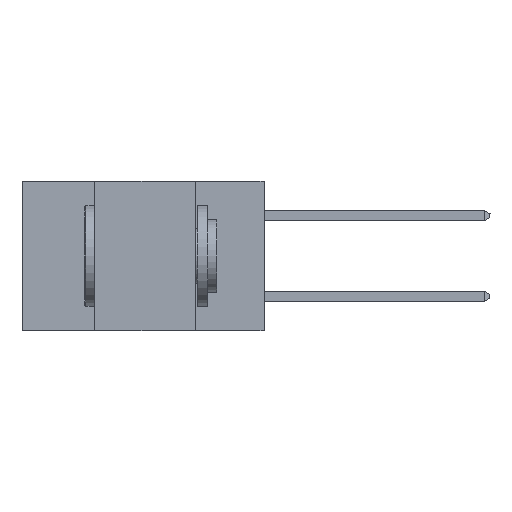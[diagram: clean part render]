
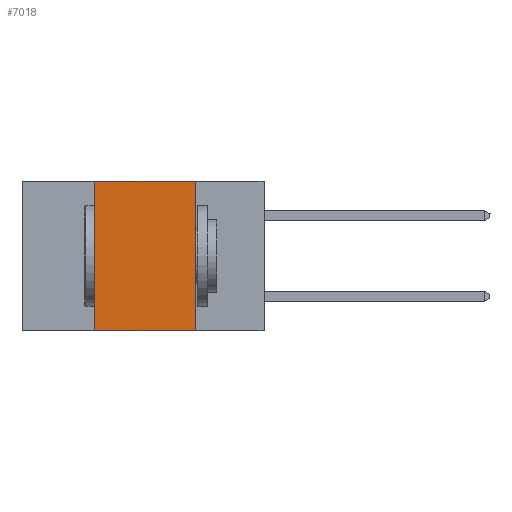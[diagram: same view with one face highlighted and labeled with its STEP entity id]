
A CAD part, left-side view. The second image highlights one B-rep face of the part: STEP entity #7018.
In plain terms, the highlighted planar face has unit normal (-1, 0, 0).
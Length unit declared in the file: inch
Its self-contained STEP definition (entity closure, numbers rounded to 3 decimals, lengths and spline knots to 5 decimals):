
#452 = VERTEX_POINT ( 'NONE', #6241 ) ;
#821 = CARTESIAN_POINT ( 'NONE',  ( 0., 0.42, 0. ) ) ;
#1814 = VECTOR ( 'NONE', #8609, 39.37008 ) ;
#2559 = DIRECTION ( 'NONE',  ( 0., 0., 1. ) ) ;
#2739 = VERTEX_POINT ( 'NONE', #3098 ) ;
#3098 = CARTESIAN_POINT ( 'NONE',  ( 0., 0.17, -0.37 ) ) ;
#3528 = EDGE_LOOP ( 'NONE', ( #12160, #8300, #13146, #19462 ) ) ;
#3588 = CARTESIAN_POINT ( 'NONE',  ( 0., 0.6, 0. ) ) ;
#6241 = CARTESIAN_POINT ( 'NONE',  ( 0., 0.42, 0. ) ) ;
#6945 = CARTESIAN_POINT ( 'NONE',  ( 0., 0.6, 0. ) ) ;
#7010 = DIRECTION ( 'NONE',  ( 1., 0., 0. ) ) ;
#7018 = ADVANCED_FACE ( 'NONE', ( #9118 ), #16418, .F. ) ;
#7103 = CARTESIAN_POINT ( 'NONE',  ( 0., 0.17, 0. ) ) ;
#7182 = LINE ( 'NONE', #19060, #18537 ) ;
#7195 = CARTESIAN_POINT ( 'NONE',  ( 0., 0.17, 0. ) ) ;
#7639 = EDGE_CURVE ( 'NONE', #452, #11667, #8620, .T. ) ;
#8300 = ORIENTED_EDGE ( 'NONE', *, *, #7639, .F. ) ;
#8609 = DIRECTION ( 'NONE',  ( 0., 0., -1. ) ) ;
#8620 = LINE ( 'NONE', #3588, #16059 ) ;
#9118 = FACE_OUTER_BOUND ( 'NONE', #3528, .T. ) ;
#9201 = VECTOR ( 'NONE', #2559, 39.37008 ) ;
#10899 = DIRECTION ( 'NONE',  ( 0., -1., 0. ) ) ;
#11667 = VERTEX_POINT ( 'NONE', #7195 ) ;
#11759 = EDGE_CURVE ( 'NONE', #14309, #452, #17639, .T. ) ;
#12160 = ORIENTED_EDGE ( 'NONE', *, *, #19548, .F. ) ;
#13059 = CARTESIAN_POINT ( 'NONE',  ( 0., 0.42, -0.37 ) ) ;
#13146 = ORIENTED_EDGE ( 'NONE', *, *, #11759, .F. ) ;
#13215 = LINE ( 'NONE', #7103, #1814 ) ;
#14309 = VERTEX_POINT ( 'NONE', #13059 ) ;
#14642 = DIRECTION ( 'NONE',  ( 0., -1., 0. ) ) ;
#14991 = EDGE_CURVE ( 'NONE', #14309, #2739, #7182, .T. ) ;
#16059 = VECTOR ( 'NONE', #14642, 39.37008 ) ;
#16418 = PLANE ( 'NONE',  #20054 ) ;
#17639 = LINE ( 'NONE', #821, #9201 ) ;
#18211 = DIRECTION ( 'NONE',  ( 0., 0., -1. ) ) ;
#18537 = VECTOR ( 'NONE', #10899, 39.37008 ) ;
#19060 = CARTESIAN_POINT ( 'NONE',  ( 0., 0.6, -0.37 ) ) ;
#19462 = ORIENTED_EDGE ( 'NONE', *, *, #14991, .T. ) ;
#19548 = EDGE_CURVE ( 'NONE', #11667, #2739, #13215, .T. ) ;
#20054 = AXIS2_PLACEMENT_3D ( 'NONE', #6945, #7010, #18211 ) ;
